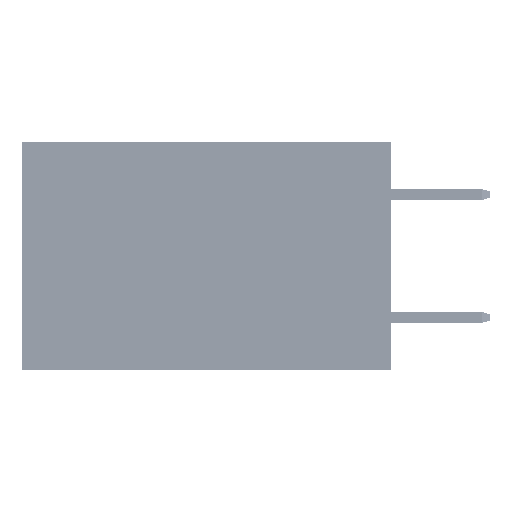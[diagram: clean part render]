
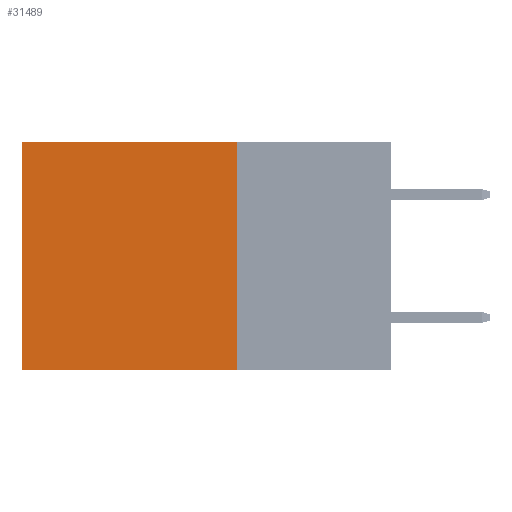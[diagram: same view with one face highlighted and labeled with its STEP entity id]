
A CAD part, left-side view. The second image highlights one B-rep face of the part: STEP entity #31489.
In plain terms, the highlighted planar face has unit normal (-1, 0, 0).
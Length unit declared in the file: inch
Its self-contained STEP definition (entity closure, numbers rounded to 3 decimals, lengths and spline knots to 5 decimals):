
#1216 = LINE ( 'NONE', #19563, #46292 ) ;
#2818 = VERTEX_POINT ( 'NONE', #47445 ) ;
#2821 = CARTESIAN_POINT ( 'NONE',  ( 0.2875, 0.25, 0. ) ) ;
#3460 = EDGE_CURVE ( 'NONE', #8323, #2818, #42564, .T. ) ;
#3580 = CARTESIAN_POINT ( 'NONE',  ( 0.2875, 0.6, 0. ) ) ;
#6172 = DIRECTION ( 'NONE',  ( 0., 0., -1. ) ) ;
#7845 = CARTESIAN_POINT ( 'NONE',  ( 0.2875, 0.25, -0.37 ) ) ;
#8124 = ORIENTED_EDGE ( 'NONE', *, *, #27806, .T. ) ;
#8323 = VERTEX_POINT ( 'NONE', #8448 ) ;
#8448 = CARTESIAN_POINT ( 'NONE',  ( 0.2875, 0.25, -0.37 ) ) ;
#17042 = DIRECTION ( 'NONE',  ( 0., 1., 0. ) ) ;
#17316 = DIRECTION ( 'NONE',  ( 0., 0., -1. ) ) ;
#18772 = LINE ( 'NONE', #46075, #32575 ) ;
#19563 = CARTESIAN_POINT ( 'NONE',  ( 0.2875, 0.25, 0. ) ) ;
#19738 = DIRECTION ( 'NONE',  ( 0., 0., -1. ) ) ;
#20061 = ORIENTED_EDGE ( 'NONE', *, *, #48070, .F. ) ;
#20200 = EDGE_LOOP ( 'NONE', ( #8124, #23598, #20061, #37828 ) ) ;
#20393 = FACE_OUTER_BOUND ( 'NONE', #20200, .T. ) ;
#21198 = VERTEX_POINT ( 'NONE', #3580 ) ;
#21509 = DIRECTION ( 'NONE',  ( 1., 0., 0. ) ) ;
#23598 = ORIENTED_EDGE ( 'NONE', *, *, #3460, .F. ) ;
#27806 = EDGE_CURVE ( 'NONE', #21198, #2818, #18772, .T. ) ;
#28320 = DIRECTION ( 'NONE',  ( 0., 1., 0. ) ) ;
#29322 = CARTESIAN_POINT ( 'NONE',  ( 0.2875, 0.25, 0. ) ) ;
#31489 = ADVANCED_FACE ( 'NONE', ( #20393 ), #45501, .F. ) ;
#32575 = VECTOR ( 'NONE', #6172, 39.37008 ) ;
#32754 = AXIS2_PLACEMENT_3D ( 'NONE', #33278, #21509, #17316 ) ;
#33278 = CARTESIAN_POINT ( 'NONE',  ( 0.2875, 0.25, 0. ) ) ;
#33479 = LINE ( 'NONE', #29322, #50359 ) ;
#37828 = ORIENTED_EDGE ( 'NONE', *, *, #45590, .T. ) ;
#39183 = VERTEX_POINT ( 'NONE', #2821 ) ;
#42564 = LINE ( 'NONE', #7845, #50114 ) ;
#45501 = PLANE ( 'NONE',  #32754 ) ;
#45590 = EDGE_CURVE ( 'NONE', #39183, #21198, #33479, .T. ) ;
#46075 = CARTESIAN_POINT ( 'NONE',  ( 0.2875, 0.6, 0. ) ) ;
#46292 = VECTOR ( 'NONE', #19738, 39.37008 ) ;
#47445 = CARTESIAN_POINT ( 'NONE',  ( 0.2875, 0.6, -0.37 ) ) ;
#48070 = EDGE_CURVE ( 'NONE', #39183, #8323, #1216, .T. ) ;
#50114 = VECTOR ( 'NONE', #28320, 39.37008 ) ;
#50359 = VECTOR ( 'NONE', #17042, 39.37008 ) ;
